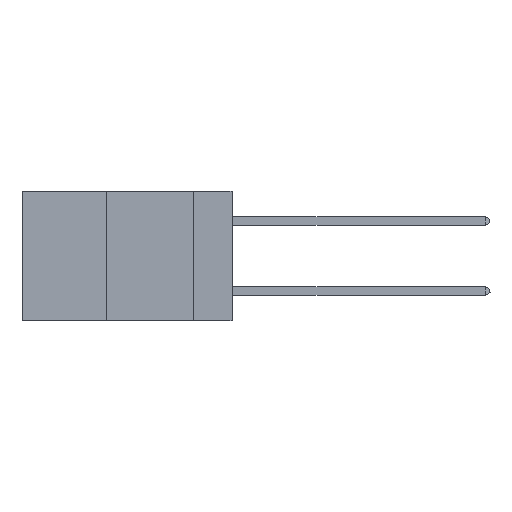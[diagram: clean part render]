
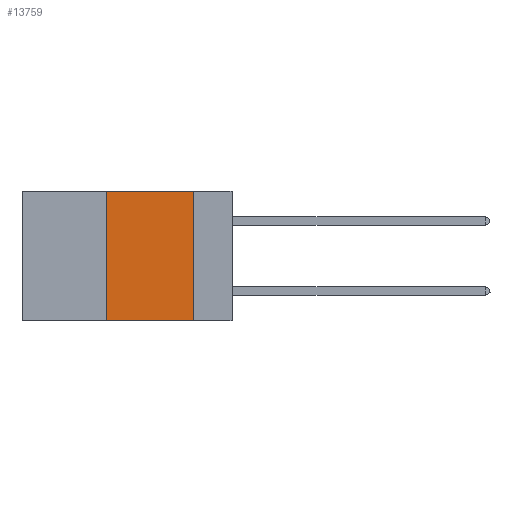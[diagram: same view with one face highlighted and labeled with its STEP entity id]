
A CAD part, left-side view. The second image highlights one B-rep face of the part: STEP entity #13759.
In plain terms, the highlighted planar face has unit normal (-1, 0, 0).
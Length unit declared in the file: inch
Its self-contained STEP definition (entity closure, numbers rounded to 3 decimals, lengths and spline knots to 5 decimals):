
#56 = DIRECTION ( 'NONE',  ( 0., 0., 1. ) ) ;
#569 = EDGE_LOOP ( 'NONE', ( #9589, #1430, #12094, #11552 ) ) ;
#1091 = DIRECTION ( 'NONE',  ( 0., -1., 0. ) ) ;
#1430 = ORIENTED_EDGE ( 'NONE', *, *, #3506, .F. ) ;
#1681 = EDGE_CURVE ( 'NONE', #11287, #1993, #2448, .T. ) ;
#1993 = VERTEX_POINT ( 'NONE', #9667 ) ;
#2358 = VECTOR ( 'NONE', #12194, 39.37008 ) ;
#2448 = LINE ( 'NONE', #2490, #4232 ) ;
#2490 = CARTESIAN_POINT ( 'NONE',  ( 0., 0.36, 0. ) ) ;
#3206 = CARTESIAN_POINT ( 'NONE',  ( 0., 0.11, 0. ) ) ;
#3215 = DIRECTION ( 'NONE',  ( 0., 0., -1. ) ) ;
#3257 = CARTESIAN_POINT ( 'NONE',  ( 0., 0.6, -0.37 ) ) ;
#3506 = EDGE_CURVE ( 'NONE', #1993, #7029, #7227, .T. ) ;
#3813 = CARTESIAN_POINT ( 'NONE',  ( 0., 0.36, -0.37 ) ) ;
#4232 = VECTOR ( 'NONE', #56, 39.37008 ) ;
#5237 = AXIS2_PLACEMENT_3D ( 'NONE', #12252, #7704, #3215 ) ;
#6555 = VECTOR ( 'NONE', #1091, 39.37008 ) ;
#7029 = VERTEX_POINT ( 'NONE', #3206 ) ;
#7124 = EDGE_CURVE ( 'NONE', #7029, #13651, #12412, .T. ) ;
#7227 = LINE ( 'NONE', #12046, #12615 ) ;
#7704 = DIRECTION ( 'NONE',  ( 1., 0., 0. ) ) ;
#9272 = CARTESIAN_POINT ( 'NONE',  ( 0., 0.11, 0. ) ) ;
#9589 = ORIENTED_EDGE ( 'NONE', *, *, #7124, .F. ) ;
#9667 = CARTESIAN_POINT ( 'NONE',  ( 0., 0.36, 0. ) ) ;
#10110 = PLANE ( 'NONE',  #5237 ) ;
#10699 = EDGE_CURVE ( 'NONE', #11287, #13651, #12835, .T. ) ;
#11287 = VERTEX_POINT ( 'NONE', #3813 ) ;
#11552 = ORIENTED_EDGE ( 'NONE', *, *, #10699, .T. ) ;
#12046 = CARTESIAN_POINT ( 'NONE',  ( 0., 0.6, 0. ) ) ;
#12094 = ORIENTED_EDGE ( 'NONE', *, *, #1681, .F. ) ;
#12194 = DIRECTION ( 'NONE',  ( 0., 0., -1. ) ) ;
#12252 = CARTESIAN_POINT ( 'NONE',  ( 0., 0.6, 0. ) ) ;
#12412 = LINE ( 'NONE', #9272, #2358 ) ;
#12615 = VECTOR ( 'NONE', #13221, 39.37008 ) ;
#12835 = LINE ( 'NONE', #3257, #6555 ) ;
#13221 = DIRECTION ( 'NONE',  ( 0., -1., 0. ) ) ;
#13651 = VERTEX_POINT ( 'NONE', #14371 ) ;
#13741 = FACE_OUTER_BOUND ( 'NONE', #569, .T. ) ;
#13759 = ADVANCED_FACE ( 'NONE', ( #13741 ), #10110, .F. ) ;
#14371 = CARTESIAN_POINT ( 'NONE',  ( 0., 0.11, -0.37 ) ) ;
